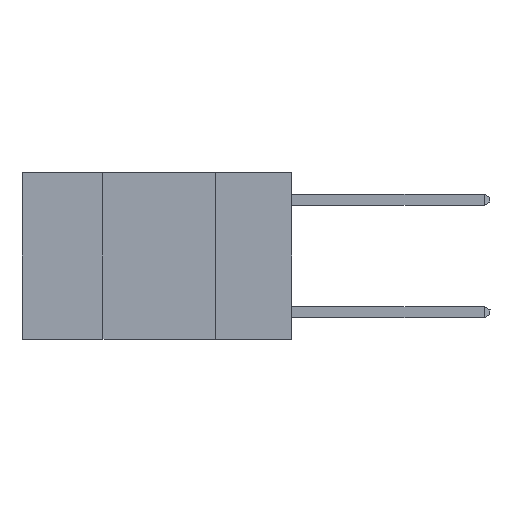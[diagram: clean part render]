
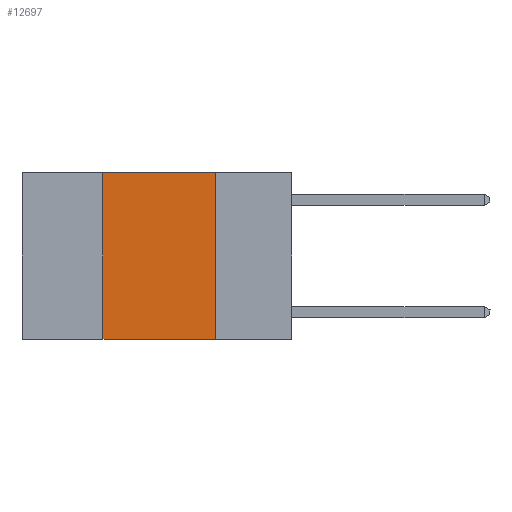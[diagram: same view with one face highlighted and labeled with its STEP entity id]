
A CAD part, left-side view. The second image highlights one B-rep face of the part: STEP entity #12697.
In plain terms, the highlighted planar face has unit normal (-1, 0, 0).
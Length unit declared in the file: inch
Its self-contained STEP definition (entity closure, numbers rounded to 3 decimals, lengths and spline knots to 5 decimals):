
#243 = LINE ( 'NONE', #269, #7988 ) ;
#269 = CARTESIAN_POINT ( 'NONE',  ( 0., 0.42, 0. ) ) ;
#629 = DIRECTION ( 'NONE',  ( 0., -1., 0. ) ) ;
#702 = VERTEX_POINT ( 'NONE', #5303 ) ;
#797 = VECTOR ( 'NONE', #629, 39.37008 ) ;
#1320 = DIRECTION ( 'NONE',  ( 0., 0., 1. ) ) ;
#1565 = VERTEX_POINT ( 'NONE', #12379 ) ;
#1678 = AXIS2_PLACEMENT_3D ( 'NONE', #10459, #11382, #5649 ) ;
#3163 = VECTOR ( 'NONE', #10240, 39.37008 ) ;
#3303 = EDGE_LOOP ( 'NONE', ( #8663, #8863, #8966, #8998 ) ) ;
#3380 = CARTESIAN_POINT ( 'NONE',  ( 0., 0.42, -0.37 ) ) ;
#3866 = LINE ( 'NONE', #5756, #797 ) ;
#4550 = EDGE_CURVE ( 'NONE', #1565, #5561, #8414, .T. ) ;
#4873 = DIRECTION ( 'NONE',  ( 0., -1., 0. ) ) ;
#5303 = CARTESIAN_POINT ( 'NONE',  ( 0., 0.42, 0. ) ) ;
#5561 = VERTEX_POINT ( 'NONE', #5769 ) ;
#5649 = DIRECTION ( 'NONE',  ( 0., 0., -1. ) ) ;
#5756 = CARTESIAN_POINT ( 'NONE',  ( 0., 0.6, -0.37 ) ) ;
#5769 = CARTESIAN_POINT ( 'NONE',  ( 0., 0.17, -0.37 ) ) ;
#5885 = EDGE_CURVE ( 'NONE', #10228, #702, #243, .T. ) ;
#6413 = CARTESIAN_POINT ( 'NONE',  ( 0., 0.17, 0. ) ) ;
#6740 = FACE_OUTER_BOUND ( 'NONE', #3303, .T. ) ;
#7898 = LINE ( 'NONE', #10674, #12553 ) ;
#7988 = VECTOR ( 'NONE', #1320, 39.37008 ) ;
#8414 = LINE ( 'NONE', #6413, #3163 ) ;
#8663 = ORIENTED_EDGE ( 'NONE', *, *, #4550, .F. ) ;
#8863 = ORIENTED_EDGE ( 'NONE', *, *, #9848, .F. ) ;
#8966 = ORIENTED_EDGE ( 'NONE', *, *, #5885, .F. ) ;
#8998 = ORIENTED_EDGE ( 'NONE', *, *, #9780, .T. ) ;
#9513 = PLANE ( 'NONE',  #1678 ) ;
#9780 = EDGE_CURVE ( 'NONE', #10228, #5561, #3866, .T. ) ;
#9848 = EDGE_CURVE ( 'NONE', #702, #1565, #7898, .T. ) ;
#10228 = VERTEX_POINT ( 'NONE', #3380 ) ;
#10240 = DIRECTION ( 'NONE',  ( 0., 0., -1. ) ) ;
#10459 = CARTESIAN_POINT ( 'NONE',  ( 0., 0.6, 0. ) ) ;
#10674 = CARTESIAN_POINT ( 'NONE',  ( 0., 0.6, 0. ) ) ;
#11382 = DIRECTION ( 'NONE',  ( 1., 0., 0. ) ) ;
#12379 = CARTESIAN_POINT ( 'NONE',  ( 0., 0.17, 0. ) ) ;
#12553 = VECTOR ( 'NONE', #4873, 39.37008 ) ;
#12697 = ADVANCED_FACE ( 'NONE', ( #6740 ), #9513, .F. ) ;
